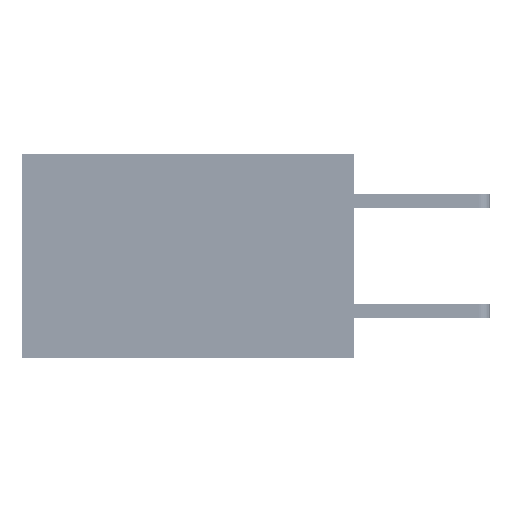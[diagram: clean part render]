
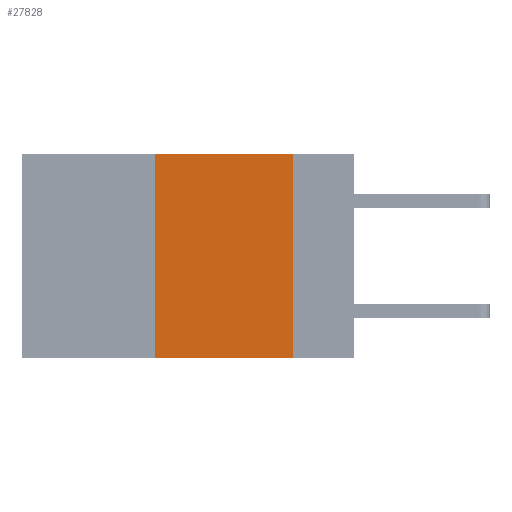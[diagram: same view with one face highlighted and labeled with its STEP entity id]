
A CAD part, left-side view. The second image highlights one B-rep face of the part: STEP entity #27828.
In plain terms, the highlighted planar face has unit normal (-1, 0, 0).
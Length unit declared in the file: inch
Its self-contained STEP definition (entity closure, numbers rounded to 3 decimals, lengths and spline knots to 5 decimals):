
#1557 = DIRECTION ( 'NONE',  ( 0., 0., -1. ) ) ;
#2627 = DIRECTION ( 'NONE',  ( 0., -1., 0. ) ) ;
#3755 = VERTEX_POINT ( 'NONE', #34238 ) ;
#4367 = DIRECTION ( 'NONE',  ( 0., -1., 0. ) ) ;
#5144 = EDGE_LOOP ( 'NONE', ( #18454, #33268, #20327, #34575 ) ) ;
#10441 = LINE ( 'NONE', #49297, #43879 ) ;
#13901 = VERTEX_POINT ( 'NONE', #18644 ) ;
#14841 = EDGE_CURVE ( 'NONE', #29261, #31453, #10441, .T. ) ;
#14991 = VECTOR ( 'NONE', #4367, 39.37008 ) ;
#15934 = FACE_OUTER_BOUND ( 'NONE', #5144, .T. ) ;
#16329 = EDGE_CURVE ( 'NONE', #13901, #3755, #34652, .T. ) ;
#16595 = VECTOR ( 'NONE', #1557, 39.37008 ) ;
#18454 = ORIENTED_EDGE ( 'NONE', *, *, #19194, .F. ) ;
#18644 = CARTESIAN_POINT ( 'NONE',  ( 0., 0.36, -0.37 ) ) ;
#19194 = EDGE_CURVE ( 'NONE', #31453, #3755, #35373, .T. ) ;
#19230 = PLANE ( 'NONE',  #48933 ) ;
#19927 = DIRECTION ( 'NONE',  ( 0., 0., 1. ) ) ;
#20327 = ORIENTED_EDGE ( 'NONE', *, *, #46522, .F. ) ;
#23031 = CARTESIAN_POINT ( 'NONE',  ( 0., 0.36, 0. ) ) ;
#26793 = DIRECTION ( 'NONE',  ( 1., 0., 0. ) ) ;
#26836 = CARTESIAN_POINT ( 'NONE',  ( 0., 0.6, -0.37 ) ) ;
#27040 = DIRECTION ( 'NONE',  ( 0., 0., -1. ) ) ;
#27828 = ADVANCED_FACE ( 'NONE', ( #15934 ), #19230, .F. ) ;
#29261 = VERTEX_POINT ( 'NONE', #23031 ) ;
#30865 = VECTOR ( 'NONE', #19927, 39.37008 ) ;
#31453 = VERTEX_POINT ( 'NONE', #34313 ) ;
#33268 = ORIENTED_EDGE ( 'NONE', *, *, #14841, .F. ) ;
#34238 = CARTESIAN_POINT ( 'NONE',  ( 0., 0.11, -0.37 ) ) ;
#34313 = CARTESIAN_POINT ( 'NONE',  ( 0., 0.11, 0. ) ) ;
#34575 = ORIENTED_EDGE ( 'NONE', *, *, #16329, .T. ) ;
#34652 = LINE ( 'NONE', #26836, #14991 ) ;
#34861 = CARTESIAN_POINT ( 'NONE',  ( 0., 0.6, 0. ) ) ;
#35373 = LINE ( 'NONE', #36124, #16595 ) ;
#36124 = CARTESIAN_POINT ( 'NONE',  ( 0., 0.11, 0. ) ) ;
#39098 = LINE ( 'NONE', #42160, #30865 ) ;
#42160 = CARTESIAN_POINT ( 'NONE',  ( 0., 0.36, 0. ) ) ;
#43879 = VECTOR ( 'NONE', #2627, 39.37008 ) ;
#46522 = EDGE_CURVE ( 'NONE', #13901, #29261, #39098, .T. ) ;
#48933 = AXIS2_PLACEMENT_3D ( 'NONE', #34861, #26793, #27040 ) ;
#49297 = CARTESIAN_POINT ( 'NONE',  ( 0., 0.6, 0. ) ) ;
